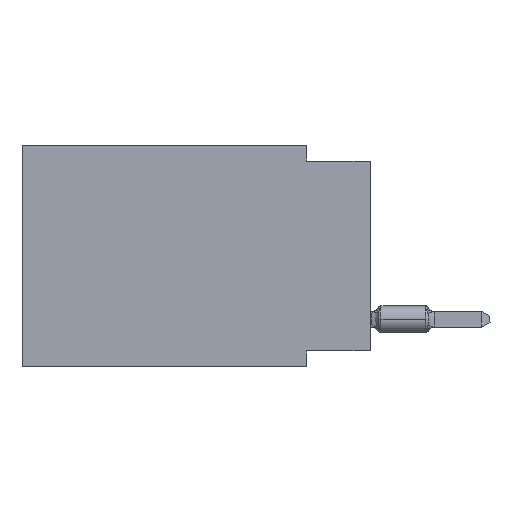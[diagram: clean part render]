
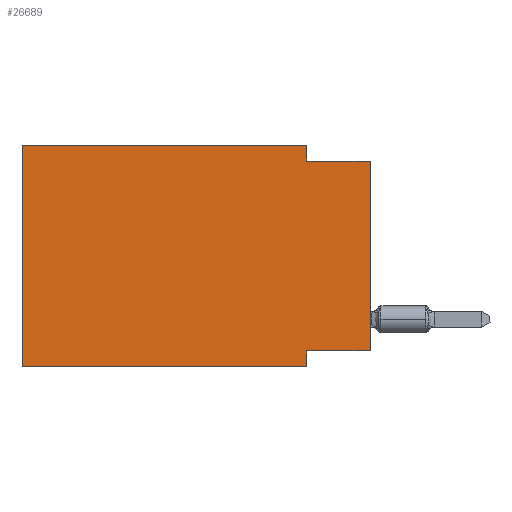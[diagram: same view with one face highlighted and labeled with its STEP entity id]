
A CAD part, left-side view. The second image highlights one B-rep face of the part: STEP entity #26689.
In plain terms, the highlighted planar face has unit normal (-1, 0, 0).
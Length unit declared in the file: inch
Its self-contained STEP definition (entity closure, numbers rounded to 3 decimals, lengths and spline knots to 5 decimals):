
#492 = LINE ( 'NONE', #29195, #36726 ) ;
#573 = VERTEX_POINT ( 'NONE', #36802 ) ;
#1014 = EDGE_CURVE ( 'NONE', #7571, #8630, #18794, .T. ) ;
#1735 = DIRECTION ( 'NONE',  ( 0., -1., 0. ) ) ;
#2634 = CARTESIAN_POINT ( 'NONE',  ( 0., 0.55, 0. ) ) ;
#2751 = LINE ( 'NONE', #20943, #19044 ) ;
#2959 = EDGE_CURVE ( 'NONE', #27481, #5444, #35779, .T. ) ;
#3618 = CARTESIAN_POINT ( 'NONE',  ( 0., 0.55, 0. ) ) ;
#3651 = CARTESIAN_POINT ( 'NONE',  ( 0., 0.55, 0. ) ) ;
#3934 = CARTESIAN_POINT ( 'NONE',  ( 0., 0.1, 0. ) ) ;
#5181 = VECTOR ( 'NONE', #17009, 39.37008 ) ;
#5444 = VERTEX_POINT ( 'NONE', #26289 ) ;
#7229 = VECTOR ( 'NONE', #9480, 39.37008 ) ;
#7388 = DIRECTION ( 'NONE',  ( 0., -1., 0. ) ) ;
#7516 = CARTESIAN_POINT ( 'NONE',  ( 0., 0.55, 0. ) ) ;
#7571 = VERTEX_POINT ( 'NONE', #3651 ) ;
#8381 = CARTESIAN_POINT ( 'NONE',  ( 0., 0., -0.025 ) ) ;
#8630 = VERTEX_POINT ( 'NONE', #3934 ) ;
#8637 = LINE ( 'NONE', #3618, #7229 ) ;
#8801 = ORIENTED_EDGE ( 'NONE', *, *, #29033, .F. ) ;
#9379 = EDGE_CURVE ( 'NONE', #11073, #28183, #20028, .T. ) ;
#9480 = DIRECTION ( 'NONE',  ( 0., 0., 1. ) ) ;
#10383 = ORIENTED_EDGE ( 'NONE', *, *, #1014, .F. ) ;
#11073 = VERTEX_POINT ( 'NONE', #20032 ) ;
#11087 = CARTESIAN_POINT ( 'NONE',  ( 0., 0., -0.025 ) ) ;
#11139 = ORIENTED_EDGE ( 'NONE', *, *, #9379, .T. ) ;
#11289 = CARTESIAN_POINT ( 'NONE',  ( 0., 0.1, 0. ) ) ;
#11576 = CARTESIAN_POINT ( 'NONE',  ( 0., 0.1, -0.325 ) ) ;
#11586 = VERTEX_POINT ( 'NONE', #29197 ) ;
#12099 = VECTOR ( 'NONE', #36910, 39.37008 ) ;
#13156 = CARTESIAN_POINT ( 'NONE',  ( 0., 0.1, -0.35 ) ) ;
#14463 = PLANE ( 'NONE',  #34718 ) ;
#14537 = ORIENTED_EDGE ( 'NONE', *, *, #32436, .F. ) ;
#15796 = ORIENTED_EDGE ( 'NONE', *, *, #30764, .F. ) ;
#15895 = VECTOR ( 'NONE', #1735, 39.37008 ) ;
#17009 = DIRECTION ( 'NONE',  ( 0., 0., 1. ) ) ;
#17840 = VECTOR ( 'NONE', #7388, 39.37008 ) ;
#18794 = LINE ( 'NONE', #7516, #17840 ) ;
#19044 = VECTOR ( 'NONE', #33650, 39.37008 ) ;
#19087 = EDGE_LOOP ( 'NONE', ( #11139, #30589, #14537, #10383, #15796, #27382, #33065, #8801 ) ) ;
#20028 = LINE ( 'NONE', #22735, #5181 ) ;
#20032 = CARTESIAN_POINT ( 'NONE',  ( 0., 0., -0.325 ) ) ;
#20943 = CARTESIAN_POINT ( 'NONE',  ( 0., 0., -0.325 ) ) ;
#22735 = CARTESIAN_POINT ( 'NONE',  ( 0., 0., 0. ) ) ;
#23414 = DIRECTION ( 'NONE',  ( 0., 0., -1. ) ) ;
#24323 = VECTOR ( 'NONE', #29065, 39.37008 ) ;
#26197 = LINE ( 'NONE', #11289, #24323 ) ;
#26289 = CARTESIAN_POINT ( 'NONE',  ( 0., 0.1, -0.35 ) ) ;
#26608 = EDGE_CURVE ( 'NONE', #573, #28183, #34508, .T. ) ;
#26689 = ADVANCED_FACE ( 'NONE', ( #33116 ), #14463, .F. ) ;
#27382 = ORIENTED_EDGE ( 'NONE', *, *, #38249, .T. ) ;
#27481 = VERTEX_POINT ( 'NONE', #11576 ) ;
#28183 = VERTEX_POINT ( 'NONE', #8381 ) ;
#29033 = EDGE_CURVE ( 'NONE', #11073, #27481, #2751, .T. ) ;
#29065 = DIRECTION ( 'NONE',  ( 0., 0., -1. ) ) ;
#29195 = CARTESIAN_POINT ( 'NONE',  ( 0., 0.55, -0.35 ) ) ;
#29197 = CARTESIAN_POINT ( 'NONE',  ( 0., 0.55, -0.35 ) ) ;
#30589 = ORIENTED_EDGE ( 'NONE', *, *, #26608, .F. ) ;
#30764 = EDGE_CURVE ( 'NONE', #11586, #7571, #8637, .T. ) ;
#32436 = EDGE_CURVE ( 'NONE', #8630, #573, #26197, .T. ) ;
#33065 = ORIENTED_EDGE ( 'NONE', *, *, #2959, .F. ) ;
#33108 = DIRECTION ( 'NONE',  ( 0., -1., 0. ) ) ;
#33116 = FACE_OUTER_BOUND ( 'NONE', #19087, .T. ) ;
#33650 = DIRECTION ( 'NONE',  ( 0., 1., 0. ) ) ;
#34508 = LINE ( 'NONE', #11087, #15895 ) ;
#34718 = AXIS2_PLACEMENT_3D ( 'NONE', #2634, #37977, #23414 ) ;
#35779 = LINE ( 'NONE', #13156, #12099 ) ;
#36726 = VECTOR ( 'NONE', #33108, 39.37008 ) ;
#36802 = CARTESIAN_POINT ( 'NONE',  ( 0., 0.1, -0.025 ) ) ;
#36910 = DIRECTION ( 'NONE',  ( 0., 0., -1. ) ) ;
#37977 = DIRECTION ( 'NONE',  ( 1., 0., 0. ) ) ;
#38249 = EDGE_CURVE ( 'NONE', #11586, #5444, #492, .T. ) ;
